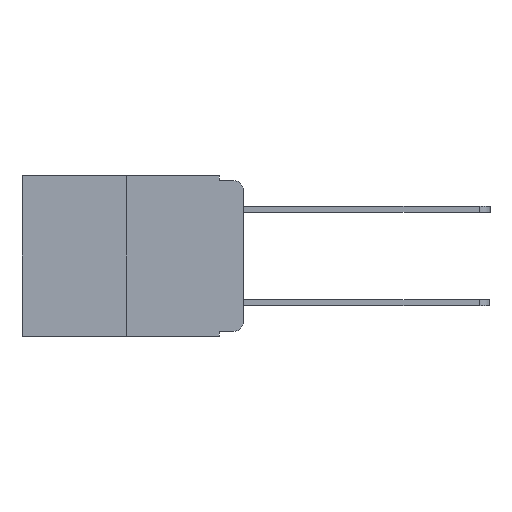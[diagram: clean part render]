
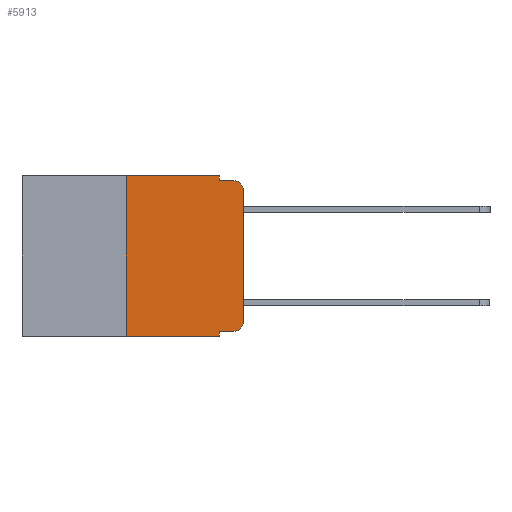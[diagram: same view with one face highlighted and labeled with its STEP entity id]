
A CAD part, left-side view. The second image highlights one B-rep face of the part: STEP entity #5913.
In plain terms, the highlighted planar face has unit normal (-1, 0, 0).
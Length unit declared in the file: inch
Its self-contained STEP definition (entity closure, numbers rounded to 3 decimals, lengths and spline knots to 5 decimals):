
#130 = CARTESIAN_POINT ( 'NONE',  ( 0., 0.473, -0.343 ) ) ;
#461 = DIRECTION ( 'NONE',  ( 0., -1., 0. ) ) ;
#1153 = LINE ( 'NONE', #20121, #6086 ) ;
#1224 = AXIS2_PLACEMENT_3D ( 'NONE', #20951, #11292, #1326 ) ;
#1245 = ORIENTED_EDGE ( 'NONE', *, *, #9597, .F. ) ;
#1301 = LINE ( 'NONE', #7634, #18276 ) ;
#1326 = DIRECTION ( 'NONE',  ( 0., 0., -1. ) ) ;
#1420 = VERTEX_POINT ( 'NONE', #19504 ) ;
#2562 = ORIENTED_EDGE ( 'NONE', *, *, #12942, .F. ) ;
#3091 = EDGE_CURVE ( 'NONE', #5534, #9941, #1153, .T. ) ;
#3331 = LINE ( 'NONE', #130, #20190 ) ;
#3758 = CARTESIAN_POINT ( 'NONE',  ( 0., 0.051, 0. ) ) ;
#3829 = CARTESIAN_POINT ( 'NONE',  ( 0., 0.02, -0.333 ) ) ;
#4045 = EDGE_CURVE ( 'NONE', #7328, #10834, #17088, .T. ) ;
#4525 = LINE ( 'NONE', #12180, #20348 ) ;
#4945 = LINE ( 'NONE', #7704, #13253 ) ;
#5249 = DIRECTION ( 'NONE',  ( 1., 0., 0. ) ) ;
#5260 = CARTESIAN_POINT ( 'NONE',  ( 0., 0.02, -0.03 ) ) ;
#5337 = LINE ( 'NONE', #3758, #13655 ) ;
#5423 = DIRECTION ( 'NONE',  ( 0., 0., -1. ) ) ;
#5534 = VERTEX_POINT ( 'NONE', #12534 ) ;
#5913 = ADVANCED_FACE ( 'NONE', ( #15787 ), #18297, .F. ) ;
#6038 = DIRECTION ( 'NONE',  ( 0., 0., 1. ) ) ;
#6086 = VECTOR ( 'NONE', #10454, 39.37008 ) ;
#6241 = EDGE_CURVE ( 'NONE', #12410, #7328, #1301, .T. ) ;
#6918 = DIRECTION ( 'NONE',  ( 0., 0., -1. ) ) ;
#7200 = ORIENTED_EDGE ( 'NONE', *, *, #16188, .T. ) ;
#7221 = VERTEX_POINT ( 'NONE', #11813 ) ;
#7328 = VERTEX_POINT ( 'NONE', #3829 ) ;
#7352 = EDGE_CURVE ( 'NONE', #12410, #12212, #4525, .T. ) ;
#7634 = CARTESIAN_POINT ( 'NONE',  ( 0., 0.051, -0.333 ) ) ;
#7703 = DIRECTION ( 'NONE',  ( 0., -1., 0. ) ) ;
#7704 = CARTESIAN_POINT ( 'NONE',  ( 0., 0.25, 0. ) ) ;
#7724 = ORIENTED_EDGE ( 'NONE', *, *, #14027, .F. ) ;
#8194 = EDGE_LOOP ( 'NONE', ( #7200, #15968, #7724, #2562, #16222, #1245, #17094, #17597, #12040, #10755 ) ) ;
#8707 = CARTESIAN_POINT ( 'NONE',  ( 0., 0.051, 0. ) ) ;
#8712 = CARTESIAN_POINT ( 'NONE',  ( 0., 0.051, -0.01 ) ) ;
#9475 = VECTOR ( 'NONE', #17776, 39.37008 ) ;
#9597 = EDGE_CURVE ( 'NONE', #14034, #5534, #4945, .T. ) ;
#9647 = CARTESIAN_POINT ( 'NONE',  ( 0., 0., -0.313 ) ) ;
#9941 = VERTEX_POINT ( 'NONE', #8707 ) ;
#10454 = DIRECTION ( 'NONE',  ( 0., -1., 0. ) ) ;
#10461 = VERTEX_POINT ( 'NONE', #18042 ) ;
#10755 = ORIENTED_EDGE ( 'NONE', *, *, #4045, .T. ) ;
#10834 = VERTEX_POINT ( 'NONE', #9647 ) ;
#11003 = EDGE_CURVE ( 'NONE', #14034, #12212, #3331, .T. ) ;
#11292 = DIRECTION ( 'NONE',  ( -1., 0., 0. ) ) ;
#11813 = CARTESIAN_POINT ( 'NONE',  ( 0., 0.02, -0.01 ) ) ;
#11843 = CARTESIAN_POINT ( 'NONE',  ( 0., 0.051, -0.343 ) ) ;
#12040 = ORIENTED_EDGE ( 'NONE', *, *, #6241, .T. ) ;
#12180 = CARTESIAN_POINT ( 'NONE',  ( 0., 0.051, 0. ) ) ;
#12212 = VERTEX_POINT ( 'NONE', #11843 ) ;
#12410 = VERTEX_POINT ( 'NONE', #20345 ) ;
#12534 = CARTESIAN_POINT ( 'NONE',  ( 0., 0.25, 0. ) ) ;
#12942 = EDGE_CURVE ( 'NONE', #9941, #1420, #5337, .T. ) ;
#13168 = CIRCLE ( 'NONE', #14431, 0.02 ) ;
#13253 = VECTOR ( 'NONE', #6038, 39.37008 ) ;
#13655 = VECTOR ( 'NONE', #5423, 39.37008 ) ;
#14027 = EDGE_CURVE ( 'NONE', #1420, #7221, #17237, .T. ) ;
#14034 = VERTEX_POINT ( 'NONE', #16943 ) ;
#14431 = AXIS2_PLACEMENT_3D ( 'NONE', #5260, #16769, #6918 ) ;
#15036 = DIRECTION ( 'NONE',  ( 0., -1., 0. ) ) ;
#15119 = EDGE_CURVE ( 'NONE', #10461, #7221, #13168, .T. ) ;
#15156 = CARTESIAN_POINT ( 'NONE',  ( 0., 0.473, 0. ) ) ;
#15787 = FACE_OUTER_BOUND ( 'NONE', #8194, .T. ) ;
#15968 = ORIENTED_EDGE ( 'NONE', *, *, #15119, .T. ) ;
#16174 = CARTESIAN_POINT ( 'NONE',  ( 0., 0., 0. ) ) ;
#16188 = EDGE_CURVE ( 'NONE', #10834, #10461, #18630, .T. ) ;
#16222 = ORIENTED_EDGE ( 'NONE', *, *, #3091, .F. ) ;
#16737 = VECTOR ( 'NONE', #461, 39.37008 ) ;
#16762 = DIRECTION ( 'NONE',  ( 0., 0., -1. ) ) ;
#16769 = DIRECTION ( 'NONE',  ( -1., 0., 0. ) ) ;
#16943 = CARTESIAN_POINT ( 'NONE',  ( 0., 0.25, -0.343 ) ) ;
#17088 = CIRCLE ( 'NONE', #1224, 0.02 ) ;
#17094 = ORIENTED_EDGE ( 'NONE', *, *, #11003, .T. ) ;
#17237 = LINE ( 'NONE', #8712, #16737 ) ;
#17597 = ORIENTED_EDGE ( 'NONE', *, *, #7352, .F. ) ;
#17776 = DIRECTION ( 'NONE',  ( 0., 0., 1. ) ) ;
#18042 = CARTESIAN_POINT ( 'NONE',  ( 0., 0., -0.03 ) ) ;
#18276 = VECTOR ( 'NONE', #7703, 39.37008 ) ;
#18297 = PLANE ( 'NONE',  #18586 ) ;
#18586 = AXIS2_PLACEMENT_3D ( 'NONE', #15156, #5249, #16762 ) ;
#18630 = LINE ( 'NONE', #16174, #9475 ) ;
#19504 = CARTESIAN_POINT ( 'NONE',  ( 0., 0.051, -0.01 ) ) ;
#20121 = CARTESIAN_POINT ( 'NONE',  ( 0., 0.473, 0. ) ) ;
#20180 = DIRECTION ( 'NONE',  ( 0., 0., -1. ) ) ;
#20190 = VECTOR ( 'NONE', #15036, 39.37008 ) ;
#20345 = CARTESIAN_POINT ( 'NONE',  ( 0., 0.051, -0.333 ) ) ;
#20348 = VECTOR ( 'NONE', #20180, 39.37008 ) ;
#20951 = CARTESIAN_POINT ( 'NONE',  ( 0., 0.02, -0.313 ) ) ;
